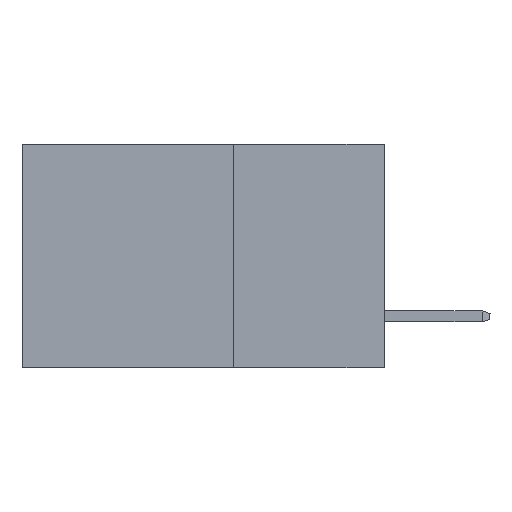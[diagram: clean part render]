
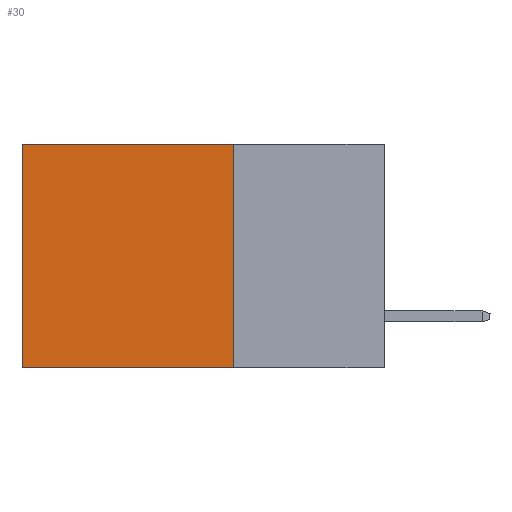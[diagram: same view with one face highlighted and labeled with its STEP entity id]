
A CAD part, left-side view. The second image highlights one B-rep face of the part: STEP entity #30.
In plain terms, the highlighted planar face has unit normal (-1, 0, 0).
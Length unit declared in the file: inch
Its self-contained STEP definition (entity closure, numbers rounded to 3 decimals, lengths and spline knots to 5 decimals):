
#30 = ADVANCED_FACE ( 'NONE', ( #3165 ), #2425, .F. ) ;
#263 = LINE ( 'NONE', #2594, #5860 ) ;
#323 = DIRECTION ( 'NONE',  ( 0., 0., -1. ) ) ;
#746 = VERTEX_POINT ( 'NONE', #1195 ) ;
#845 = VECTOR ( 'NONE', #5300, 39.37008 ) ;
#955 = VERTEX_POINT ( 'NONE', #6622 ) ;
#1195 = CARTESIAN_POINT ( 'NONE',  ( 0.2615, 0.6, 0. ) ) ;
#1203 = CARTESIAN_POINT ( 'NONE',  ( 0.2615, 0.25, -0.37 ) ) ;
#1226 = DIRECTION ( 'NONE',  ( 1., 0., 0. ) ) ;
#2425 = PLANE ( 'NONE',  #9934 ) ;
#2594 = CARTESIAN_POINT ( 'NONE',  ( 0.2615, 0.6, -0.37 ) ) ;
#2609 = CARTESIAN_POINT ( 'NONE',  ( 0.2615, 0.25, 0. ) ) ;
#3148 = EDGE_CURVE ( 'NONE', #746, #5780, #263, .T. ) ;
#3165 = FACE_OUTER_BOUND ( 'NONE', #3267, .T. ) ;
#3267 = EDGE_LOOP ( 'NONE', ( #7326, #9689, #4822, #8408 ) ) ;
#3747 = VERTEX_POINT ( 'NONE', #10915 ) ;
#3912 = EDGE_CURVE ( 'NONE', #3747, #746, #7643, .T. ) ;
#4255 = DIRECTION ( 'NONE',  ( 0., 0., -1. ) ) ;
#4822 = ORIENTED_EDGE ( 'NONE', *, *, #6537, .F. ) ;
#5300 = DIRECTION ( 'NONE',  ( 0., 1., 0. ) ) ;
#5434 = EDGE_CURVE ( 'NONE', #955, #5780, #6169, .T. ) ;
#5575 = VECTOR ( 'NONE', #10541, 39.37008 ) ;
#5780 = VERTEX_POINT ( 'NONE', #7496 ) ;
#5860 = VECTOR ( 'NONE', #323, 39.37008 ) ;
#6169 = LINE ( 'NONE', #1203, #845 ) ;
#6524 = VECTOR ( 'NONE', #12724, 39.37008 ) ;
#6537 = EDGE_CURVE ( 'NONE', #3747, #955, #10479, .T. ) ;
#6622 = CARTESIAN_POINT ( 'NONE',  ( 0.2615, 0.25, -0.37 ) ) ;
#7326 = ORIENTED_EDGE ( 'NONE', *, *, #3148, .T. ) ;
#7496 = CARTESIAN_POINT ( 'NONE',  ( 0.2615, 0.6, -0.37 ) ) ;
#7643 = LINE ( 'NONE', #2609, #6524 ) ;
#8408 = ORIENTED_EDGE ( 'NONE', *, *, #3912, .T. ) ;
#9689 = ORIENTED_EDGE ( 'NONE', *, *, #5434, .F. ) ;
#9934 = AXIS2_PLACEMENT_3D ( 'NONE', #11537, #1226, #4255 ) ;
#10479 = LINE ( 'NONE', #12493, #5575 ) ;
#10541 = DIRECTION ( 'NONE',  ( 0., 0., -1. ) ) ;
#10915 = CARTESIAN_POINT ( 'NONE',  ( 0.2615, 0.25, 0. ) ) ;
#11537 = CARTESIAN_POINT ( 'NONE',  ( 0.2615, 0.25, -0.37 ) ) ;
#12493 = CARTESIAN_POINT ( 'NONE',  ( 0.2615, 0.25, -0.37 ) ) ;
#12724 = DIRECTION ( 'NONE',  ( 0., 1., 0. ) ) ;
